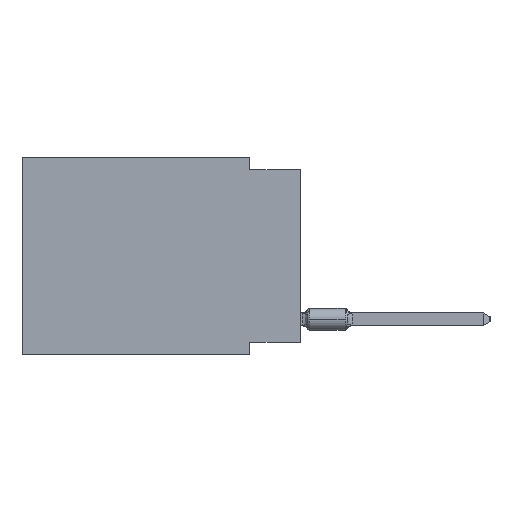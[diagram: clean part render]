
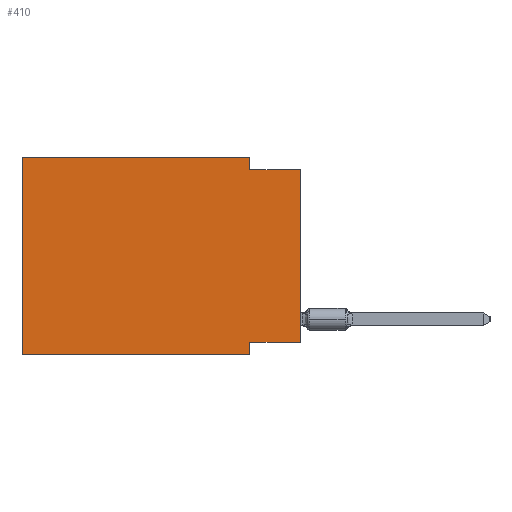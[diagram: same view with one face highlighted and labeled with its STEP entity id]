
A CAD part, left-side view. The second image highlights one B-rep face of the part: STEP entity #410.
In plain terms, the highlighted planar face has unit normal (-1, 0, 0).
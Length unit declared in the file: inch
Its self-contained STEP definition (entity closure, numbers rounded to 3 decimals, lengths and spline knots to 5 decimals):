
#257 = VERTEX_POINT ( 'NONE', #44569 ) ;
#334 = ORIENTED_EDGE ( 'NONE', *, *, #54698, .F. ) ;
#410 = ADVANCED_FACE ( 'NONE', ( #50160 ), #11874, .F. ) ;
#534 = LINE ( 'NONE', #21780, #18598 ) ;
#1392 = EDGE_CURVE ( 'NONE', #16923, #7347, #19713, .T. ) ;
#1559 = DIRECTION ( 'NONE',  ( 0., -1., 0. ) ) ;
#2145 = ORIENTED_EDGE ( 'NONE', *, *, #19511, .F. ) ;
#5447 = ORIENTED_EDGE ( 'NONE', *, *, #31096, .F. ) ;
#6307 = CARTESIAN_POINT ( 'NONE',  ( 0., 0.55, -0.39 ) ) ;
#7331 = DIRECTION ( 'NONE',  ( 0., -1., 0. ) ) ;
#7347 = VERTEX_POINT ( 'NONE', #17251 ) ;
#7669 = DIRECTION ( 'NONE',  ( 0., 0., -1. ) ) ;
#8623 = CARTESIAN_POINT ( 'NONE',  ( 0., 0., 0. ) ) ;
#10194 = EDGE_LOOP ( 'NONE', ( #26845, #5447, #334, #12938, #2145, #26374, #29325, #39286 ) ) ;
#11874 = PLANE ( 'NONE',  #39179 ) ;
#12938 = ORIENTED_EDGE ( 'NONE', *, *, #25954, .F. ) ;
#14184 = LINE ( 'NONE', #40132, #20232 ) ;
#14713 = DIRECTION ( 'NONE',  ( 0., 1., 0. ) ) ;
#15257 = VECTOR ( 'NONE', #7331, 39.37008 ) ;
#15505 = VERTEX_POINT ( 'NONE', #33082 ) ;
#15726 = LINE ( 'NONE', #54815, #15257 ) ;
#15819 = CARTESIAN_POINT ( 'NONE',  ( 0., 0., -0.365 ) ) ;
#15944 = LINE ( 'NONE', #8623, #41860 ) ;
#15980 = VECTOR ( 'NONE', #46618, 39.37008 ) ;
#16923 = VERTEX_POINT ( 'NONE', #48954 ) ;
#17251 = CARTESIAN_POINT ( 'NONE',  ( 0., 0.1, -0.365 ) ) ;
#18598 = VECTOR ( 'NONE', #48321, 39.37008 ) ;
#19097 = LINE ( 'NONE', #36425, #19121 ) ;
#19121 = VECTOR ( 'NONE', #22752, 39.37008 ) ;
#19511 = EDGE_CURVE ( 'NONE', #32619, #26020, #14184, .T. ) ;
#19713 = LINE ( 'NONE', #15819, #49967 ) ;
#20232 = VECTOR ( 'NONE', #22823, 39.37008 ) ;
#21780 = CARTESIAN_POINT ( 'NONE',  ( 0., 0., -0.025 ) ) ;
#22075 = EDGE_CURVE ( 'NONE', #7347, #44770, #38240, .T. ) ;
#22267 = VECTOR ( 'NONE', #1559, 39.37008 ) ;
#22558 = CARTESIAN_POINT ( 'NONE',  ( 0., 0.55, -0.39 ) ) ;
#22752 = DIRECTION ( 'NONE',  ( 0., 0., -1. ) ) ;
#22823 = DIRECTION ( 'NONE',  ( 0., 0., 1. ) ) ;
#23020 = CARTESIAN_POINT ( 'NONE',  ( 0., 0.1, -0.39 ) ) ;
#23838 = CARTESIAN_POINT ( 'NONE',  ( 0., 0.55, 0. ) ) ;
#25954 = EDGE_CURVE ( 'NONE', #26020, #15505, #15726, .T. ) ;
#26020 = VERTEX_POINT ( 'NONE', #23838 ) ;
#26374 = ORIENTED_EDGE ( 'NONE', *, *, #43285, .T. ) ;
#26845 = ORIENTED_EDGE ( 'NONE', *, *, #42576, .T. ) ;
#28922 = CARTESIAN_POINT ( 'NONE',  ( 0., 0.55, 0. ) ) ;
#29325 = ORIENTED_EDGE ( 'NONE', *, *, #22075, .F. ) ;
#30295 = VERTEX_POINT ( 'NONE', #46465 ) ;
#31096 = EDGE_CURVE ( 'NONE', #30295, #257, #534, .T. ) ;
#32619 = VERTEX_POINT ( 'NONE', #22558 ) ;
#33082 = CARTESIAN_POINT ( 'NONE',  ( 0., 0.1, 0. ) ) ;
#35369 = LINE ( 'NONE', #6307, #22267 ) ;
#36425 = CARTESIAN_POINT ( 'NONE',  ( 0., 0.1, 0. ) ) ;
#38240 = LINE ( 'NONE', #46887, #15980 ) ;
#39179 = AXIS2_PLACEMENT_3D ( 'NONE', #28922, #45948, #7669 ) ;
#39286 = ORIENTED_EDGE ( 'NONE', *, *, #1392, .F. ) ;
#40132 = CARTESIAN_POINT ( 'NONE',  ( 0., 0.55, 0. ) ) ;
#41629 = DIRECTION ( 'NONE',  ( 0., 0., 1. ) ) ;
#41860 = VECTOR ( 'NONE', #41629, 39.37008 ) ;
#42576 = EDGE_CURVE ( 'NONE', #16923, #257, #15944, .T. ) ;
#43285 = EDGE_CURVE ( 'NONE', #32619, #44770, #35369, .T. ) ;
#44569 = CARTESIAN_POINT ( 'NONE',  ( 0., 0., -0.025 ) ) ;
#44770 = VERTEX_POINT ( 'NONE', #23020 ) ;
#45948 = DIRECTION ( 'NONE',  ( 1., 0., 0. ) ) ;
#46465 = CARTESIAN_POINT ( 'NONE',  ( 0., 0.1, -0.025 ) ) ;
#46618 = DIRECTION ( 'NONE',  ( 0., 0., -1. ) ) ;
#46887 = CARTESIAN_POINT ( 'NONE',  ( 0., 0.1, -0.39 ) ) ;
#48321 = DIRECTION ( 'NONE',  ( 0., -1., 0. ) ) ;
#48954 = CARTESIAN_POINT ( 'NONE',  ( 0., 0., -0.365 ) ) ;
#49967 = VECTOR ( 'NONE', #14713, 39.37008 ) ;
#50160 = FACE_OUTER_BOUND ( 'NONE', #10194, .T. ) ;
#54698 = EDGE_CURVE ( 'NONE', #15505, #30295, #19097, .T. ) ;
#54815 = CARTESIAN_POINT ( 'NONE',  ( 0., 0.55, 0. ) ) ;
